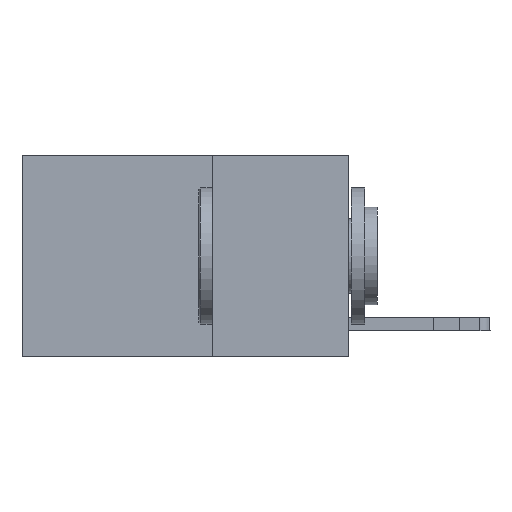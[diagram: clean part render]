
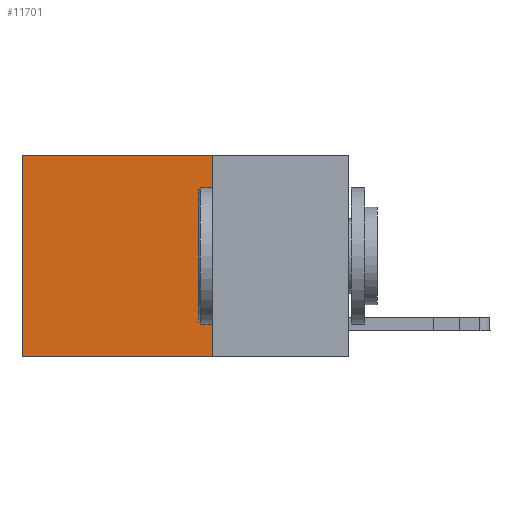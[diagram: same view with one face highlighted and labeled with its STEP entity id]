
A CAD part, left-side view. The second image highlights one B-rep face of the part: STEP entity #11701.
In plain terms, the highlighted planar face has unit normal (-1, 0, 0).
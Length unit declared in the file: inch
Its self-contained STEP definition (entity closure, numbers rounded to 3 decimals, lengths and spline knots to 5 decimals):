
#643 = CARTESIAN_POINT ( 'NONE',  ( 0.2625, 0.25, -0.37 ) ) ;
#844 = EDGE_CURVE ( 'NONE', #7739, #1936, #9316, .T. ) ;
#955 = CARTESIAN_POINT ( 'NONE',  ( 0.2625, 0.25, 0. ) ) ;
#1359 = CARTESIAN_POINT ( 'NONE',  ( 0.2625, 0.25, -0.37 ) ) ;
#1470 = ORIENTED_EDGE ( 'NONE', *, *, #2629, .F. ) ;
#1578 = ORIENTED_EDGE ( 'NONE', *, *, #10041, .T. ) ;
#1732 = PLANE ( 'NONE',  #2688 ) ;
#1936 = VERTEX_POINT ( 'NONE', #8187 ) ;
#2383 = DIRECTION ( 'NONE',  ( 0., 1., 0. ) ) ;
#2629 = EDGE_CURVE ( 'NONE', #4380, #7739, #8558, .T. ) ;
#2688 = AXIS2_PLACEMENT_3D ( 'NONE', #5578, #9471, #7806 ) ;
#3339 = LINE ( 'NONE', #7192, #7488 ) ;
#4380 = VERTEX_POINT ( 'NONE', #6568 ) ;
#4684 = EDGE_LOOP ( 'NONE', ( #12485, #10170, #1470, #1578 ) ) ;
#5578 = CARTESIAN_POINT ( 'NONE',  ( 0.2625, 0.25, 0. ) ) ;
#5678 = DIRECTION ( 'NONE',  ( 0., 0., -1. ) ) ;
#6193 = CARTESIAN_POINT ( 'NONE',  ( 0.2625, 0.6, 0. ) ) ;
#6568 = CARTESIAN_POINT ( 'NONE',  ( 0.2625, 0.25, 0. ) ) ;
#6982 = CARTESIAN_POINT ( 'NONE',  ( 0.2625, 0.6, 0. ) ) ;
#7192 = CARTESIAN_POINT ( 'NONE',  ( 0.2625, 0.25, 0. ) ) ;
#7488 = VECTOR ( 'NONE', #2383, 39.37008 ) ;
#7739 = VERTEX_POINT ( 'NONE', #1359 ) ;
#7806 = DIRECTION ( 'NONE',  ( 0., 0., -1. ) ) ;
#8187 = CARTESIAN_POINT ( 'NONE',  ( 0.2625, 0.6, -0.37 ) ) ;
#8436 = DIRECTION ( 'NONE',  ( 0., 1., 0. ) ) ;
#8558 = LINE ( 'NONE', #955, #12172 ) ;
#8931 = EDGE_CURVE ( 'NONE', #10011, #1936, #9853, .T. ) ;
#9041 = VECTOR ( 'NONE', #9916, 39.37008 ) ;
#9316 = LINE ( 'NONE', #643, #9358 ) ;
#9358 = VECTOR ( 'NONE', #8436, 39.37008 ) ;
#9471 = DIRECTION ( 'NONE',  ( 1., 0., 0. ) ) ;
#9853 = LINE ( 'NONE', #6982, #9041 ) ;
#9916 = DIRECTION ( 'NONE',  ( 0., 0., -1. ) ) ;
#10011 = VERTEX_POINT ( 'NONE', #6193 ) ;
#10041 = EDGE_CURVE ( 'NONE', #4380, #10011, #3339, .T. ) ;
#10170 = ORIENTED_EDGE ( 'NONE', *, *, #844, .F. ) ;
#11355 = FACE_OUTER_BOUND ( 'NONE', #4684, .T. ) ;
#11701 = ADVANCED_FACE ( 'NONE', ( #11355 ), #1732, .F. ) ;
#12172 = VECTOR ( 'NONE', #5678, 39.37008 ) ;
#12485 = ORIENTED_EDGE ( 'NONE', *, *, #8931, .T. ) ;
